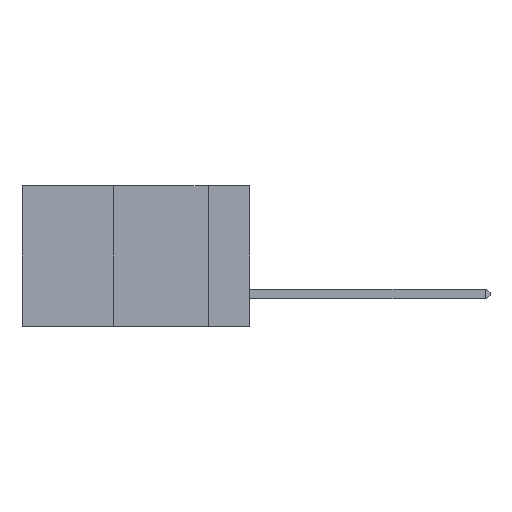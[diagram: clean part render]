
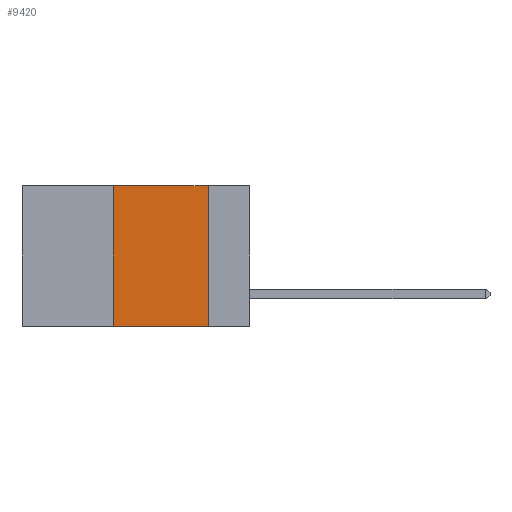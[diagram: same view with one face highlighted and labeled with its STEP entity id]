
A CAD part, left-side view. The second image highlights one B-rep face of the part: STEP entity #9420.
In plain terms, the highlighted planar face has unit normal (-1, 0, 0).
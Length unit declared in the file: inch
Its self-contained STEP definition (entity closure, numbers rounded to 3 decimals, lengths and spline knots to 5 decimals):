
#110 = VERTEX_POINT ( 'NONE', #584 ) ;
#384 = DIRECTION ( 'NONE',  ( 0., 0., 1. ) ) ;
#399 = CARTESIAN_POINT ( 'NONE',  ( 0., 0.36, 0. ) ) ;
#584 = CARTESIAN_POINT ( 'NONE',  ( 0., 0.11, -0.37 ) ) ;
#920 = VECTOR ( 'NONE', #1945, 39.37008 ) ;
#972 = EDGE_CURVE ( 'NONE', #4725, #2843, #1252, .T. ) ;
#1252 = LINE ( 'NONE', #2518, #6448 ) ;
#1945 = DIRECTION ( 'NONE',  ( 0., 0., -1. ) ) ;
#2307 = VECTOR ( 'NONE', #384, 39.37008 ) ;
#2518 = CARTESIAN_POINT ( 'NONE',  ( 0., 0.6, 0. ) ) ;
#2843 = VERTEX_POINT ( 'NONE', #3422 ) ;
#2878 = CARTESIAN_POINT ( 'NONE',  ( 0., 0.11, 0. ) ) ;
#3112 = EDGE_CURVE ( 'NONE', #4316, #4725, #4614, .T. ) ;
#3422 = CARTESIAN_POINT ( 'NONE',  ( 0., 0.11, 0. ) ) ;
#3564 = LINE ( 'NONE', #2878, #920 ) ;
#3939 = CARTESIAN_POINT ( 'NONE',  ( 0., 0.36, 0. ) ) ;
#4007 = CARTESIAN_POINT ( 'NONE',  ( 0., 0.6, 0. ) ) ;
#4162 = ORIENTED_EDGE ( 'NONE', *, *, #3112, .F. ) ;
#4176 = ORIENTED_EDGE ( 'NONE', *, *, #10169, .T. ) ;
#4316 = VERTEX_POINT ( 'NONE', #6375 ) ;
#4614 = LINE ( 'NONE', #399, #2307 ) ;
#4725 = VERTEX_POINT ( 'NONE', #3939 ) ;
#4819 = ORIENTED_EDGE ( 'NONE', *, *, #9319, .F. ) ;
#4975 = PLANE ( 'NONE',  #5808 ) ;
#5060 = ORIENTED_EDGE ( 'NONE', *, *, #972, .F. ) ;
#5808 = AXIS2_PLACEMENT_3D ( 'NONE', #4007, #11541, #5934 ) ;
#5934 = DIRECTION ( 'NONE',  ( 0., 0., -1. ) ) ;
#6375 = CARTESIAN_POINT ( 'NONE',  ( 0., 0.36, -0.37 ) ) ;
#6448 = VECTOR ( 'NONE', #9293, 39.37008 ) ;
#7293 = VECTOR ( 'NONE', #7970, 39.37008 ) ;
#7462 = FACE_OUTER_BOUND ( 'NONE', #11517, .T. ) ;
#7970 = DIRECTION ( 'NONE',  ( 0., -1., 0. ) ) ;
#8945 = CARTESIAN_POINT ( 'NONE',  ( 0., 0.6, -0.37 ) ) ;
#9254 = LINE ( 'NONE', #8945, #7293 ) ;
#9293 = DIRECTION ( 'NONE',  ( 0., -1., 0. ) ) ;
#9319 = EDGE_CURVE ( 'NONE', #2843, #110, #3564, .T. ) ;
#9420 = ADVANCED_FACE ( 'NONE', ( #7462 ), #4975, .F. ) ;
#10169 = EDGE_CURVE ( 'NONE', #4316, #110, #9254, .T. ) ;
#11517 = EDGE_LOOP ( 'NONE', ( #4819, #5060, #4162, #4176 ) ) ;
#11541 = DIRECTION ( 'NONE',  ( 1., 0., 0. ) ) ;
